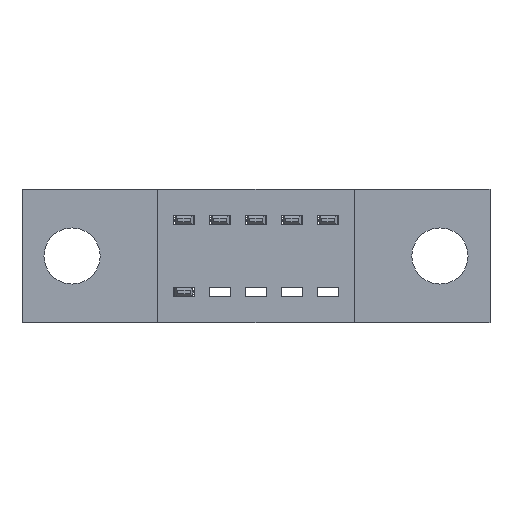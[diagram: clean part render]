
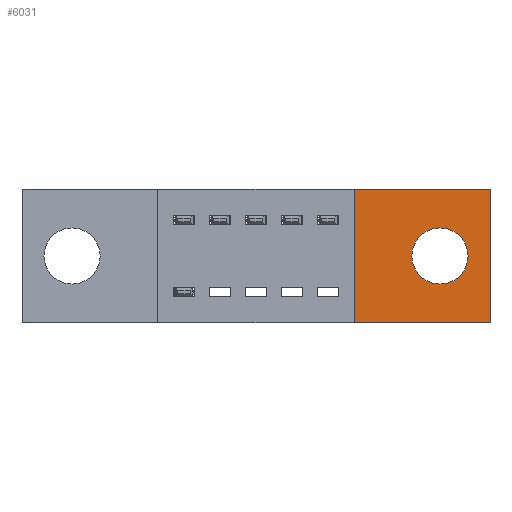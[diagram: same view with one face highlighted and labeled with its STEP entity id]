
A CAD part, front view. The second image highlights one B-rep face of the part: STEP entity #6031.
In plain terms, the highlighted planar face has unit normal (0, -1, 0).
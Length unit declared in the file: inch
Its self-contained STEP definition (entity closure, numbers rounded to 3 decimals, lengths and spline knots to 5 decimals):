
#60 = VERTEX_POINT ( 'NONE', #6500 ) ;
#409 = CIRCLE ( 'NONE', #6451, 0.078 ) ;
#557 = FACE_OUTER_BOUND ( 'NONE', #3214, .T. ) ;
#676 = CARTESIAN_POINT ( 'NONE',  ( 0., 0., -0.37 ) ) ;
#808 = EDGE_CURVE ( 'NONE', #2118, #1546, #6472, .T. ) ;
#853 = CARTESIAN_POINT ( 'NONE',  ( 1.161, 0., -0.107 ) ) ;
#865 = AXIS2_PLACEMENT_3D ( 'NONE', #1772, #3123, #2731 ) ;
#892 = EDGE_LOOP ( 'NONE', ( #1964, #3715 ) ) ;
#929 = AXIS2_PLACEMENT_3D ( 'NONE', #1675, #1833, #1622 ) ;
#1070 = DIRECTION ( 'NONE',  ( 0., 0., -1. ) ) ;
#1121 = EDGE_CURVE ( 'NONE', #1546, #2118, #409, .T. ) ;
#1147 = ORIENTED_EDGE ( 'NONE', *, *, #5298, .F. ) ;
#1166 = CARTESIAN_POINT ( 'NONE',  ( 1.161, 0., -0.185 ) ) ;
#1209 = CARTESIAN_POINT ( 'NONE',  ( 1.3, 0., 0. ) ) ;
#1336 = ORIENTED_EDGE ( 'NONE', *, *, #6099, .F. ) ;
#1394 = VECTOR ( 'NONE', #1070, 39.37008 ) ;
#1546 = VERTEX_POINT ( 'NONE', #853 ) ;
#1619 = VECTOR ( 'NONE', #6471, 39.37008 ) ;
#1622 = DIRECTION ( 'NONE',  ( 0., 0., -1. ) ) ;
#1638 = PLANE ( 'NONE',  #929 ) ;
#1675 = CARTESIAN_POINT ( 'NONE',  ( 0., 0., -0.37 ) ) ;
#1772 = CARTESIAN_POINT ( 'NONE',  ( 1.161, 0., -0.185 ) ) ;
#1833 = DIRECTION ( 'NONE',  ( 0., -1., 0. ) ) ;
#1883 = DIRECTION ( 'NONE',  ( -1., 0., 0. ) ) ;
#1964 = ORIENTED_EDGE ( 'NONE', *, *, #1121, .T. ) ;
#2094 = LINE ( 'NONE', #676, #6629 ) ;
#2117 = FACE_BOUND ( 'NONE', #892, .T. ) ;
#2118 = VERTEX_POINT ( 'NONE', #2721 ) ;
#2215 = VERTEX_POINT ( 'NONE', #6822 ) ;
#2721 = CARTESIAN_POINT ( 'NONE',  ( 1.161, 0., -0.263 ) ) ;
#2731 = DIRECTION ( 'NONE',  ( 0., 0., -1. ) ) ;
#2785 = VERTEX_POINT ( 'NONE', #5647 ) ;
#2946 = DIRECTION ( 'NONE',  ( 0., 0., -1. ) ) ;
#3077 = EDGE_CURVE ( 'NONE', #60, #2215, #6383, .T. ) ;
#3123 = DIRECTION ( 'NONE',  ( 0., 1., 0. ) ) ;
#3214 = EDGE_LOOP ( 'NONE', ( #1147, #4337, #1336, #6110 ) ) ;
#3715 = ORIENTED_EDGE ( 'NONE', *, *, #808, .T. ) ;
#3820 = CARTESIAN_POINT ( 'NONE',  ( 1.3, 0., -0.37 ) ) ;
#4217 = VECTOR ( 'NONE', #7264, 39.37008 ) ;
#4337 = ORIENTED_EDGE ( 'NONE', *, *, #7432, .F. ) ;
#4484 = VERTEX_POINT ( 'NONE', #3820 ) ;
#4975 = LINE ( 'NONE', #1209, #1394 ) ;
#5298 = EDGE_CURVE ( 'NONE', #2785, #60, #5830, .T. ) ;
#5647 = CARTESIAN_POINT ( 'NONE',  ( 0.923, 0., -0.37 ) ) ;
#5830 = LINE ( 'NONE', #7477, #4217 ) ;
#6031 = ADVANCED_FACE ( 'NONE', ( #2117, #557 ), #1638, .T. ) ;
#6099 = EDGE_CURVE ( 'NONE', #2215, #4484, #4975, .T. ) ;
#6110 = ORIENTED_EDGE ( 'NONE', *, *, #3077, .F. ) ;
#6383 = LINE ( 'NONE', #7175, #1619 ) ;
#6451 = AXIS2_PLACEMENT_3D ( 'NONE', #1166, #7295, #2946 ) ;
#6471 = DIRECTION ( 'NONE',  ( 1., 0., 0. ) ) ;
#6472 = CIRCLE ( 'NONE', #865, 0.078 ) ;
#6500 = CARTESIAN_POINT ( 'NONE',  ( 0.923, 0., 0. ) ) ;
#6629 = VECTOR ( 'NONE', #1883, 39.37008 ) ;
#6822 = CARTESIAN_POINT ( 'NONE',  ( 1.3, 0., 0. ) ) ;
#7175 = CARTESIAN_POINT ( 'NONE',  ( 0., 0., 0. ) ) ;
#7264 = DIRECTION ( 'NONE',  ( 0., 0., 1. ) ) ;
#7295 = DIRECTION ( 'NONE',  ( 0., 1., 0. ) ) ;
#7432 = EDGE_CURVE ( 'NONE', #4484, #2785, #2094, .T. ) ;
#7477 = CARTESIAN_POINT ( 'NONE',  ( 0.923, 0., -0.37 ) ) ;
